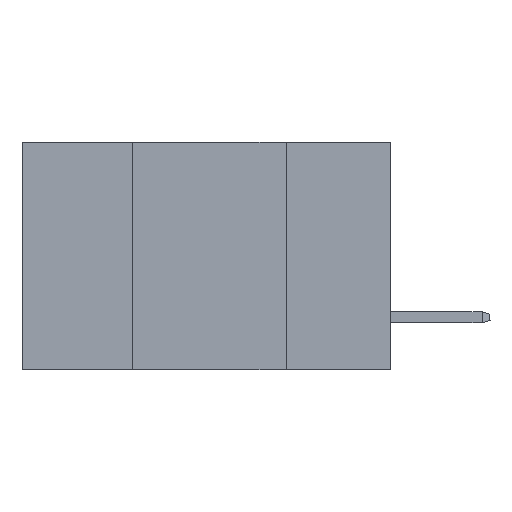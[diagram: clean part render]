
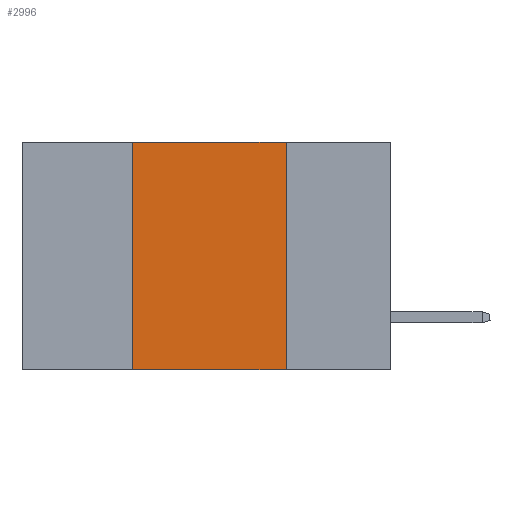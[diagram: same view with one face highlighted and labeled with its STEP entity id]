
A CAD part, left-side view. The second image highlights one B-rep face of the part: STEP entity #2996.
In plain terms, the highlighted planar face has unit normal (-1, 0, 0).
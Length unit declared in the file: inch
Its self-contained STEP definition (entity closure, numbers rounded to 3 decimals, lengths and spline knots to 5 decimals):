
#1172 = LINE ( 'NONE', #26697, #17562 ) ;
#1299 = VERTEX_POINT ( 'NONE', #38431 ) ;
#1674 = CARTESIAN_POINT ( 'NONE',  ( 0., 0.17, 0. ) ) ;
#2996 = ADVANCED_FACE ( 'NONE', ( #23656 ), #15852, .F. ) ;
#4858 = EDGE_LOOP ( 'NONE', ( #13987, #15325, #13761, #37699 ) ) ;
#5299 = LINE ( 'NONE', #35812, #38034 ) ;
#6266 = VERTEX_POINT ( 'NONE', #37261 ) ;
#12081 = CARTESIAN_POINT ( 'NONE',  ( 0., 0.6, 0. ) ) ;
#13761 = ORIENTED_EDGE ( 'NONE', *, *, #32315, .F. ) ;
#13987 = ORIENTED_EDGE ( 'NONE', *, *, #27984, .F. ) ;
#15325 = ORIENTED_EDGE ( 'NONE', *, *, #30951, .F. ) ;
#15852 = PLANE ( 'NONE',  #31457 ) ;
#17524 = DIRECTION ( 'NONE',  ( 0., 0., -1. ) ) ;
#17562 = VECTOR ( 'NONE', #29863, 39.37008 ) ;
#17771 = VERTEX_POINT ( 'NONE', #40872 ) ;
#19434 = VECTOR ( 'NONE', #17524, 39.37008 ) ;
#20566 = VECTOR ( 'NONE', #23825, 39.37008 ) ;
#20937 = EDGE_CURVE ( 'NONE', #17771, #1299, #1172, .T. ) ;
#21242 = CARTESIAN_POINT ( 'NONE',  ( 0., 0.42, 0. ) ) ;
#23656 = FACE_OUTER_BOUND ( 'NONE', #4858, .T. ) ;
#23825 = DIRECTION ( 'NONE',  ( 0., 0., 1. ) ) ;
#26697 = CARTESIAN_POINT ( 'NONE',  ( 0., 0.6, -0.37 ) ) ;
#27984 = EDGE_CURVE ( 'NONE', #6266, #1299, #31320, .T. ) ;
#29863 = DIRECTION ( 'NONE',  ( 0., -1., 0. ) ) ;
#30951 = EDGE_CURVE ( 'NONE', #36553, #6266, #5299, .T. ) ;
#31320 = LINE ( 'NONE', #1674, #19434 ) ;
#31457 = AXIS2_PLACEMENT_3D ( 'NONE', #12081, #34234, #34362 ) ;
#32315 = EDGE_CURVE ( 'NONE', #17771, #36553, #36380, .T. ) ;
#34234 = DIRECTION ( 'NONE',  ( 1., 0., 0. ) ) ;
#34362 = DIRECTION ( 'NONE',  ( 0., 0., -1. ) ) ;
#35812 = CARTESIAN_POINT ( 'NONE',  ( 0., 0.6, 0. ) ) ;
#36380 = LINE ( 'NONE', #39211, #20566 ) ;
#36553 = VERTEX_POINT ( 'NONE', #21242 ) ;
#37261 = CARTESIAN_POINT ( 'NONE',  ( 0., 0.17, 0. ) ) ;
#37699 = ORIENTED_EDGE ( 'NONE', *, *, #20937, .T. ) ;
#38034 = VECTOR ( 'NONE', #39488, 39.37008 ) ;
#38431 = CARTESIAN_POINT ( 'NONE',  ( 0., 0.17, -0.37 ) ) ;
#39211 = CARTESIAN_POINT ( 'NONE',  ( 0., 0.42, 0. ) ) ;
#39488 = DIRECTION ( 'NONE',  ( 0., -1., 0. ) ) ;
#40872 = CARTESIAN_POINT ( 'NONE',  ( 0., 0.42, -0.37 ) ) ;
